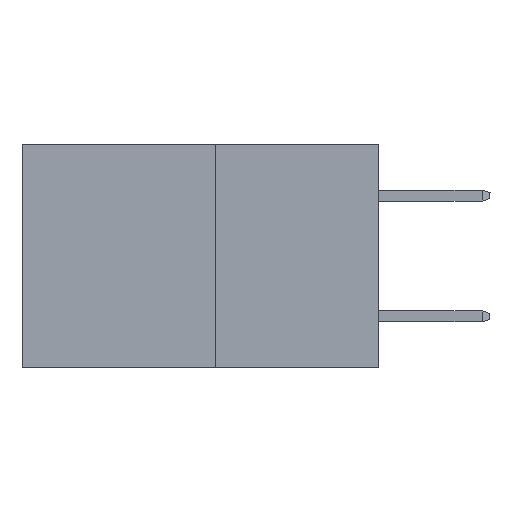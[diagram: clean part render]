
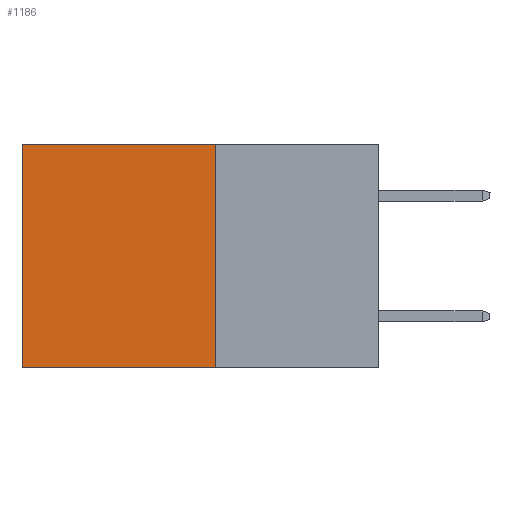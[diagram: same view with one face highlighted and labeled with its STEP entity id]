
A CAD part, left-side view. The second image highlights one B-rep face of the part: STEP entity #1186.
In plain terms, the highlighted planar face has unit normal (-1, 0, 0).
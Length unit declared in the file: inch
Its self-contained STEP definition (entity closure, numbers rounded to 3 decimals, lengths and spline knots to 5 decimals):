
#78 = CARTESIAN_POINT ( 'NONE',  ( 0.277, 0.27, 0. ) ) ;
#194 = DIRECTION ( 'NONE',  ( 0., 1., 0. ) ) ;
#878 = VECTOR ( 'NONE', #5841, 39.37008 ) ;
#1095 = LINE ( 'NONE', #78, #878 ) ;
#1186 = ADVANCED_FACE ( 'NONE', ( #3420 ), #4005, .F. ) ;
#1261 = CARTESIAN_POINT ( 'NONE',  ( 0.277, 0.27, -0.37 ) ) ;
#1703 = VERTEX_POINT ( 'NONE', #4206 ) ;
#1758 = EDGE_CURVE ( 'NONE', #7459, #1703, #1095, .T. ) ;
#1898 = CARTESIAN_POINT ( 'NONE',  ( 0.277, 0.27, 0. ) ) ;
#2471 = LINE ( 'NONE', #6426, #7573 ) ;
#2692 = EDGE_CURVE ( 'NONE', #1703, #7564, #2471, .T. ) ;
#2878 = ORIENTED_EDGE ( 'NONE', *, *, #6282, .F. ) ;
#3200 = CARTESIAN_POINT ( 'NONE',  ( 0.277, 0.27, -0.37 ) ) ;
#3420 = FACE_OUTER_BOUND ( 'NONE', #5607, .T. ) ;
#4005 = PLANE ( 'NONE',  #6524 ) ;
#4206 = CARTESIAN_POINT ( 'NONE',  ( 0.277, 0.59, 0. ) ) ;
#4595 = VECTOR ( 'NONE', #194, 39.37008 ) ;
#4603 = LINE ( 'NONE', #1261, #8130 ) ;
#4837 = ORIENTED_EDGE ( 'NONE', *, *, #5813, .F. ) ;
#4987 = CARTESIAN_POINT ( 'NONE',  ( 0.277, 0.27, -0.37 ) ) ;
#5524 = DIRECTION ( 'NONE',  ( 0., 0., -1. ) ) ;
#5607 = EDGE_LOOP ( 'NONE', ( #8133, #2878, #4837, #8337 ) ) ;
#5813 = EDGE_CURVE ( 'NONE', #7459, #5999, #4603, .T. ) ;
#5841 = DIRECTION ( 'NONE',  ( 0., 1., 0. ) ) ;
#5848 = CARTESIAN_POINT ( 'NONE',  ( 0.277, 0.27, -0.37 ) ) ;
#5999 = VERTEX_POINT ( 'NONE', #4987 ) ;
#6282 = EDGE_CURVE ( 'NONE', #5999, #7564, #6379, .T. ) ;
#6379 = LINE ( 'NONE', #5848, #4595 ) ;
#6426 = CARTESIAN_POINT ( 'NONE',  ( 0.277, 0.59, -0.37 ) ) ;
#6524 = AXIS2_PLACEMENT_3D ( 'NONE', #3200, #8647, #6529 ) ;
#6529 = DIRECTION ( 'NONE',  ( 0., 0., -1. ) ) ;
#7459 = VERTEX_POINT ( 'NONE', #1898 ) ;
#7564 = VERTEX_POINT ( 'NONE', #8836 ) ;
#7573 = VECTOR ( 'NONE', #8900, 39.37008 ) ;
#8130 = VECTOR ( 'NONE', #5524, 39.37008 ) ;
#8133 = ORIENTED_EDGE ( 'NONE', *, *, #2692, .T. ) ;
#8337 = ORIENTED_EDGE ( 'NONE', *, *, #1758, .T. ) ;
#8647 = DIRECTION ( 'NONE',  ( 1., 0., 0. ) ) ;
#8836 = CARTESIAN_POINT ( 'NONE',  ( 0.277, 0.59, -0.37 ) ) ;
#8900 = DIRECTION ( 'NONE',  ( 0., 0., -1. ) ) ;
